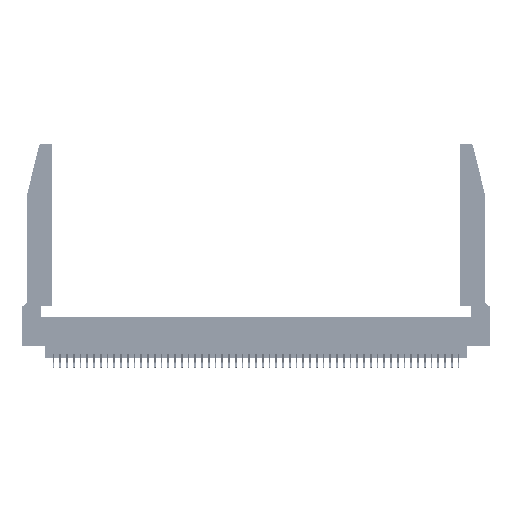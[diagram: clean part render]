
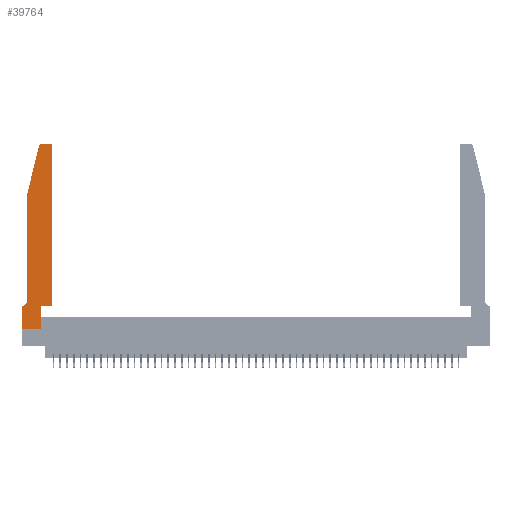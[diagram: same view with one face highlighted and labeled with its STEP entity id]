
A CAD part, top view. The second image highlights one B-rep face of the part: STEP entity #39764.
In plain terms, the highlighted planar face has unit normal (0, 0, 1).
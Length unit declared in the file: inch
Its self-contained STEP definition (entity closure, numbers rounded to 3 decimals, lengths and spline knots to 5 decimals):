
#94 = VECTOR ( 'NONE', #21016, 39.37008 ) ;
#860 = ORIENTED_EDGE ( 'NONE', *, *, #31820, .T. ) ;
#2664 = CARTESIAN_POINT ( 'NONE',  ( 0.4505, 0.35, 0.37 ) ) ;
#2942 = VECTOR ( 'NONE', #10612, 39.37008 ) ;
#4147 = CARTESIAN_POINT ( 'NONE',  ( 0.4505, 2.72, 0.37 ) ) ;
#5366 = CARTESIAN_POINT ( 'NONE',  ( 0.4505, 0.35, 0.37 ) ) ;
#5588 = ORIENTED_EDGE ( 'NONE', *, *, #47772, .T. ) ;
#5604 = CARTESIAN_POINT ( 'NONE',  ( 0., 0., 0.37 ) ) ;
#6590 = VECTOR ( 'NONE', #13490, 39.37008 ) ;
#7806 = LINE ( 'NONE', #12621, #28574 ) ;
#8031 = AXIS2_PLACEMENT_3D ( 'NONE', #43661, #20388, #47536 ) ;
#8699 = DIRECTION ( 'NONE',  ( 0., 1., 0. ) ) ;
#10190 = ORIENTED_EDGE ( 'NONE', *, *, #48923, .T. ) ;
#10293 = CARTESIAN_POINT ( 'NONE',  ( 0., 0., 0.37 ) ) ;
#10612 = DIRECTION ( 'NONE',  ( 0., -1., 0. ) ) ;
#10937 = EDGE_CURVE ( 'NONE', #22380, #23119, #16418, .T. ) ;
#11929 = LINE ( 'NONE', #12031, #45416 ) ;
#12031 = CARTESIAN_POINT ( 'NONE',  ( 0.0755, 0.35, 0.37 ) ) ;
#12393 = CIRCLE ( 'NONE', #8031, 0.03 ) ;
#12609 = VERTEX_POINT ( 'NONE', #5366 ) ;
#12621 = CARTESIAN_POINT ( 'NONE',  ( 0.4505, 0.35, 0.37 ) ) ;
#13326 = EDGE_CURVE ( 'NONE', #21949, #45170, #25343, .T. ) ;
#13490 = DIRECTION ( 'NONE',  ( 0., -1., 0. ) ) ;
#13578 = ORIENTED_EDGE ( 'NONE', *, *, #20430, .T. ) ;
#14144 = ORIENTED_EDGE ( 'NONE', *, *, #38205, .T. ) ;
#14740 = DIRECTION ( 'NONE',  ( -0.239, -0.971, 0. ) ) ;
#16418 = CIRCLE ( 'NONE', #17324, 0.07 ) ;
#16734 = VERTEX_POINT ( 'NONE', #20963 ) ;
#17152 = CARTESIAN_POINT ( 'NONE',  ( 0.4205, 2.72, 0.37 ) ) ;
#17324 = AXIS2_PLACEMENT_3D ( 'NONE', #18875, #46046, #22810 ) ;
#17890 = ORIENTED_EDGE ( 'NONE', *, *, #10937, .T. ) ;
#18127 = EDGE_CURVE ( 'NONE', #25201, #26842, #32267, .T. ) ;
#18492 = CARTESIAN_POINT ( 'NONE',  ( 0.0755, 2., 0.37 ) ) ;
#18875 = CARTESIAN_POINT ( 'NONE',  ( 0.0055, 0.42, 0.37 ) ) ;
#18944 = EDGE_CURVE ( 'NONE', #43385, #46742, #12393, .T. ) ;
#19708 = EDGE_CURVE ( 'NONE', #45170, #43385, #40369, .T. ) ;
#20388 = DIRECTION ( 'NONE',  ( 0., 0., 1. ) ) ;
#20430 = EDGE_CURVE ( 'NONE', #26842, #27289, #27610, .T. ) ;
#20509 = CARTESIAN_POINT ( 'NONE',  ( 0.2865, 0., 0.37 ) ) ;
#20963 = CARTESIAN_POINT ( 'NONE',  ( 0.2865, 0.35, 0.37 ) ) ;
#21016 = DIRECTION ( 'NONE',  ( -1., 0., 0. ) ) ;
#21089 = DIRECTION ( 'NONE',  ( 1., 0., 0. ) ) ;
#21949 = VERTEX_POINT ( 'NONE', #4147 ) ;
#22004 = CARTESIAN_POINT ( 'NONE',  ( 0., 0., 0.37 ) ) ;
#22149 = VECTOR ( 'NONE', #14740, 39.37008 ) ;
#22184 = CARTESIAN_POINT ( 'NONE',  ( 0., 0.35, 0.37 ) ) ;
#22337 = DIRECTION ( 'NONE',  ( 1., 0., 0. ) ) ;
#22350 = EDGE_CURVE ( 'NONE', #46809, #22380, #23726, .T. ) ;
#22380 = VERTEX_POINT ( 'NONE', #37913 ) ;
#22737 = EDGE_CURVE ( 'NONE', #12609, #21949, #7806, .T. ) ;
#22810 = DIRECTION ( 'NONE',  ( -1., 0., 0. ) ) ;
#23119 = VERTEX_POINT ( 'NONE', #30898 ) ;
#23726 = LINE ( 'NONE', #34023, #2942 ) ;
#25201 = VERTEX_POINT ( 'NONE', #39234 ) ;
#25343 = CIRCLE ( 'NONE', #37641, 0.03 ) ;
#25857 = DIRECTION ( 'NONE',  ( 0., 1., 0. ) ) ;
#26092 = DIRECTION ( 'NONE',  ( 1., 0., 0. ) ) ;
#26842 = VERTEX_POINT ( 'NONE', #10293 ) ;
#26899 = ORIENTED_EDGE ( 'NONE', *, *, #18127, .T. ) ;
#27242 = LINE ( 'NONE', #2664, #45426 ) ;
#27289 = VERTEX_POINT ( 'NONE', #20509 ) ;
#27610 = LINE ( 'NONE', #22004, #37954 ) ;
#27668 = LINE ( 'NONE', #49094, #48276 ) ;
#28574 = VECTOR ( 'NONE', #8699, 39.37008 ) ;
#28905 = ORIENTED_EDGE ( 'NONE', *, *, #22737, .T. ) ;
#29935 = FACE_OUTER_BOUND ( 'NONE', #31558, .T. ) ;
#30898 = CARTESIAN_POINT ( 'NONE',  ( 0.0055, 0.35, 0.37 ) ) ;
#31558 = EDGE_LOOP ( 'NONE', ( #49176, #33400, #860, #32650, #17890, #5588, #26899, #13578, #10190, #14144, #28905, #32104 ) ) ;
#31820 = EDGE_CURVE ( 'NONE', #46742, #46809, #43987, .T. ) ;
#32104 = ORIENTED_EDGE ( 'NONE', *, *, #13326, .T. ) ;
#32267 = LINE ( 'NONE', #5604, #6590 ) ;
#32650 = ORIENTED_EDGE ( 'NONE', *, *, #22350, .T. ) ;
#33400 = ORIENTED_EDGE ( 'NONE', *, *, #18944, .T. ) ;
#33780 = PLANE ( 'NONE',  #45642 ) ;
#34023 = CARTESIAN_POINT ( 'NONE',  ( 0.0755, 2., 0.37 ) ) ;
#37547 = CARTESIAN_POINT ( 'NONE',  ( 0.0755, 2., 0.37 ) ) ;
#37641 = AXIS2_PLACEMENT_3D ( 'NONE', #17152, #44343, #21089 ) ;
#37913 = CARTESIAN_POINT ( 'NONE',  ( 0.0755, 0.42, 0.37 ) ) ;
#37954 = VECTOR ( 'NONE', #41552, 39.37008 ) ;
#38205 = EDGE_CURVE ( 'NONE', #16734, #12609, #27242, .T. ) ;
#39234 = CARTESIAN_POINT ( 'NONE',  ( 0., 0.35, 0.37 ) ) ;
#39299 = DIRECTION ( 'NONE',  ( -1., 0., 0. ) ) ;
#39764 = ADVANCED_FACE ( 'NONE', ( #29935 ), #33780, .T. ) ;
#40369 = LINE ( 'NONE', #48161, #94 ) ;
#41552 = DIRECTION ( 'NONE',  ( 1., 0., 0. ) ) ;
#43385 = VERTEX_POINT ( 'NONE', #47728 ) ;
#43661 = CARTESIAN_POINT ( 'NONE',  ( 0.284, 2.72, 0.37 ) ) ;
#43987 = LINE ( 'NONE', #18492, #22149 ) ;
#44343 = DIRECTION ( 'NONE',  ( 0., 0., 1. ) ) ;
#44796 = CARTESIAN_POINT ( 'NONE',  ( 0.25487, 2.72718, 0.37 ) ) ;
#45170 = VERTEX_POINT ( 'NONE', #46419 ) ;
#45416 = VECTOR ( 'NONE', #39299, 39.37008 ) ;
#45426 = VECTOR ( 'NONE', #22337, 39.37008 ) ;
#45642 = AXIS2_PLACEMENT_3D ( 'NONE', #22184, #49331, #26092 ) ;
#46046 = DIRECTION ( 'NONE',  ( 0., 0., -1. ) ) ;
#46419 = CARTESIAN_POINT ( 'NONE',  ( 0.4205, 2.75, 0.37 ) ) ;
#46742 = VERTEX_POINT ( 'NONE', #44796 ) ;
#46809 = VERTEX_POINT ( 'NONE', #37547 ) ;
#47536 = DIRECTION ( 'NONE',  ( 1., 0., 0. ) ) ;
#47728 = CARTESIAN_POINT ( 'NONE',  ( 0.284, 2.75, 0.37 ) ) ;
#47772 = EDGE_CURVE ( 'NONE', #23119, #25201, #11929, .T. ) ;
#48161 = CARTESIAN_POINT ( 'NONE',  ( 0.2605, 2.75, 0.37 ) ) ;
#48276 = VECTOR ( 'NONE', #25857, 39.37008 ) ;
#48923 = EDGE_CURVE ( 'NONE', #27289, #16734, #27668, .T. ) ;
#49094 = CARTESIAN_POINT ( 'NONE',  ( 0.2865, 0.35, 0.37 ) ) ;
#49176 = ORIENTED_EDGE ( 'NONE', *, *, #19708, .T. ) ;
#49331 = DIRECTION ( 'NONE',  ( 0., 0., 1. ) ) ;
